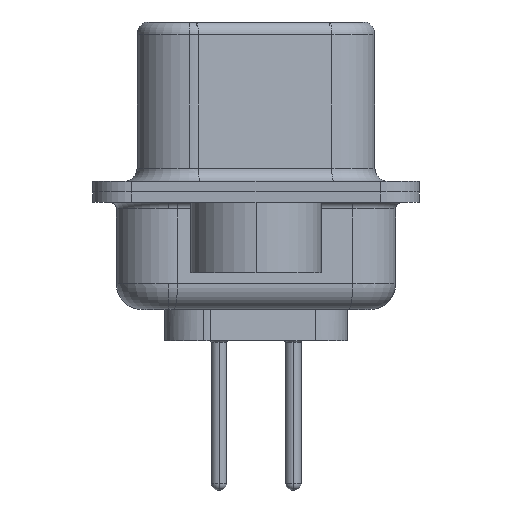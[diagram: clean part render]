
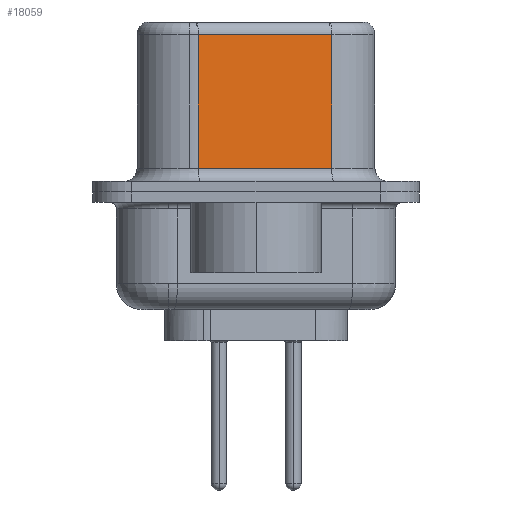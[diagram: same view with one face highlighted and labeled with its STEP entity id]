
A CAD part, left-side view. The second image highlights one B-rep face of the part: STEP entity #18059.
In plain terms, the highlighted planar face has unit normal (-0.985, -0.174, 0).
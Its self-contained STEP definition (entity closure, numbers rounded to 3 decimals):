
#13 = LINE ( 'NONE', #15438, #20052 ) ;
#146 = DIRECTION ( 'NONE',  ( 0.985, 0.174, 0. ) ) ;
#771 = DIRECTION ( 'NONE',  ( 0.174, -0.985, 0. ) ) ;
#1455 = CARTESIAN_POINT ( 'NONE',  ( 4.58, -2.897, 6.02 ) ) ;
#1574 = DIRECTION ( 'NONE',  ( -0.174, 0.985, 0. ) ) ;
#2026 = CARTESIAN_POINT ( 'NONE',  ( 4.58, -2.897, 6.52 ) ) ;
#2195 = EDGE_LOOP ( 'NONE', ( #23406, #11838, #3130, #24954 ) ) ;
#2576 = VECTOR ( 'NONE', #1574, 1000. ) ;
#3130 = ORIENTED_EDGE ( 'NONE', *, *, #18096, .T. ) ;
#3637 = VECTOR ( 'NONE', #9876, 1000. ) ;
#3685 = FACE_OUTER_BOUND ( 'NONE', #2195, .T. ) ;
#3812 = PLANE ( 'NONE',  #6305 ) ;
#5288 = EDGE_CURVE ( 'NONE', #23715, #8259, #23943, .T. ) ;
#6305 = AXIS2_PLACEMENT_3D ( 'NONE', #2026, #146, #19260 ) ;
#7781 = EDGE_CURVE ( 'NONE', #11489, #8259, #13911, .T. ) ;
#7955 = CARTESIAN_POINT ( 'NONE',  ( 4.58, -2.897, 0.9 ) ) ;
#8259 = VERTEX_POINT ( 'NONE', #7955 ) ;
#9876 = DIRECTION ( 'NONE',  ( 0., 0., -1. ) ) ;
#11489 = VERTEX_POINT ( 'NONE', #21129 ) ;
#11567 = CARTESIAN_POINT ( 'NONE',  ( 3.68, 2.203, 0.9 ) ) ;
#11669 = EDGE_CURVE ( 'NONE', #11489, #16535, #20966, .T. ) ;
#11838 = ORIENTED_EDGE ( 'NONE', *, *, #11669, .T. ) ;
#13911 = LINE ( 'NONE', #16049, #3637 ) ;
#15438 = CARTESIAN_POINT ( 'NONE',  ( 3.68, 2.203, 6.52 ) ) ;
#16049 = CARTESIAN_POINT ( 'NONE',  ( 4.58, -2.897, 6.52 ) ) ;
#16535 = VERTEX_POINT ( 'NONE', #19348 ) ;
#18059 = ADVANCED_FACE ( 'NONE', ( #3685 ), #3812, .F. ) ;
#18096 = EDGE_CURVE ( 'NONE', #16535, #23715, #13, .T. ) ;
#19260 = DIRECTION ( 'NONE',  ( -0.174, 0.985, 0. ) ) ;
#19348 = CARTESIAN_POINT ( 'NONE',  ( 3.68, 2.203, 6.02 ) ) ;
#20052 = VECTOR ( 'NONE', #23191, 1000. ) ;
#20966 = LINE ( 'NONE', #1455, #2576 ) ;
#21129 = CARTESIAN_POINT ( 'NONE',  ( 4.58, -2.897, 6.02 ) ) ;
#23191 = DIRECTION ( 'NONE',  ( 0., 0., -1. ) ) ;
#23406 = ORIENTED_EDGE ( 'NONE', *, *, #7781, .F. ) ;
#23715 = VERTEX_POINT ( 'NONE', #11567 ) ;
#23943 = LINE ( 'NONE', #24064, #24200 ) ;
#24064 = CARTESIAN_POINT ( 'NONE',  ( 4.58, -2.897, 0.9 ) ) ;
#24200 = VECTOR ( 'NONE', #771, 1000. ) ;
#24954 = ORIENTED_EDGE ( 'NONE', *, *, #5288, .T. ) ;
